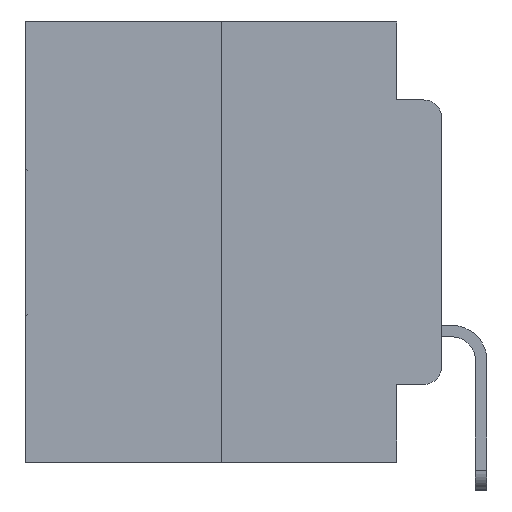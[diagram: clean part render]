
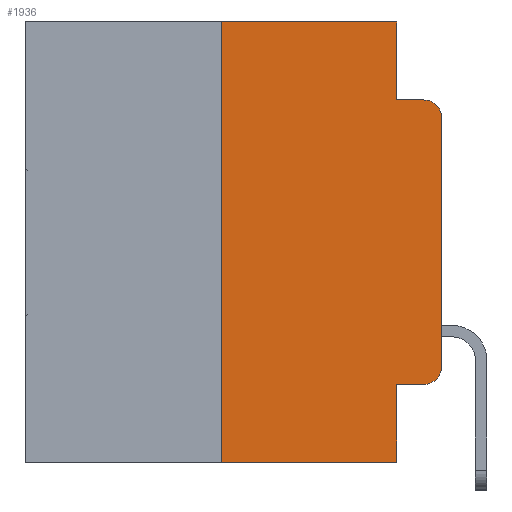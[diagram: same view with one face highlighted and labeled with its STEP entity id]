
A CAD part, left-side view. The second image highlights one B-rep face of the part: STEP entity #1936.
In plain terms, the highlighted planar face has unit normal (-1, 0, 0).
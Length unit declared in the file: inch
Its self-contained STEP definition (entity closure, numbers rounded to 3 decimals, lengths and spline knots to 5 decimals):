
#555 = VERTEX_POINT ( 'NONE', #10674 ) ;
#632 = DIRECTION ( 'NONE',  ( 0., 0., 1. ) ) ;
#837 = DIRECTION ( 'NONE',  ( 0., 0., -1. ) ) ;
#1332 = AXIS2_PLACEMENT_3D ( 'NONE', #7820, #5532, #3255 ) ;
#1486 = DIRECTION ( 'NONE',  ( 0., 0., -1. ) ) ;
#1936 = ADVANCED_FACE ( 'NONE', ( #3103 ), #12876, .F. ) ;
#2161 = AXIS2_PLACEMENT_3D ( 'NONE', #9277, #5025, #837 ) ;
#2241 = ORIENTED_EDGE ( 'NONE', *, *, #6701, .F. ) ;
#2416 = EDGE_CURVE ( 'NONE', #3343, #555, #13606, .T. ) ;
#2468 = DIRECTION ( 'NONE',  ( 0., 0., -1. ) ) ;
#2716 = DIRECTION ( 'NONE',  ( 0., -1., 0. ) ) ;
#3103 = FACE_OUTER_BOUND ( 'NONE', #27822, .T. ) ;
#3255 = DIRECTION ( 'NONE',  ( 0., 0., -1. ) ) ;
#3343 = VERTEX_POINT ( 'NONE', #7509 ) ;
#3593 = DIRECTION ( 'NONE',  ( 0., -1., 0. ) ) ;
#4059 = VECTOR ( 'NONE', #19508, 39.37008 ) ;
#4067 = DIRECTION ( 'NONE',  ( 1., 0., 0. ) ) ;
#4178 = CARTESIAN_POINT ( 'NONE',  ( 0., 0.051, -0.0885 ) ) ;
#4420 = ORIENTED_EDGE ( 'NONE', *, *, #24878, .T. ) ;
#4927 = EDGE_CURVE ( 'NONE', #12223, #23504, #20556, .T. ) ;
#4953 = VERTEX_POINT ( 'NONE', #5848 ) ;
#5025 = DIRECTION ( 'NONE',  ( -1., 0., 0. ) ) ;
#5071 = DIRECTION ( 'NONE',  ( 0., 0., 1. ) ) ;
#5532 = DIRECTION ( 'NONE',  ( -1., 0., 0. ) ) ;
#5848 = CARTESIAN_POINT ( 'NONE',  ( 0., 0.25, -0.5 ) ) ;
#5850 = LINE ( 'NONE', #15894, #25465 ) ;
#6072 = DIRECTION ( 'NONE',  ( 0., 0., -1. ) ) ;
#6505 = LINE ( 'NONE', #15685, #25771 ) ;
#6598 = VECTOR ( 'NONE', #16787, 39.37008 ) ;
#6701 = EDGE_CURVE ( 'NONE', #25876, #19956, #26361, .T. ) ;
#6724 = ORIENTED_EDGE ( 'NONE', *, *, #12757, .F. ) ;
#7311 = VECTOR ( 'NONE', #3593, 39.37008 ) ;
#7509 = CARTESIAN_POINT ( 'NONE',  ( 0., 0.02, -0.4115 ) ) ;
#7820 = CARTESIAN_POINT ( 'NONE',  ( 0., 0.02, -0.3915 ) ) ;
#8266 = CARTESIAN_POINT ( 'NONE',  ( 0., 0.25, 0. ) ) ;
#8915 = CARTESIAN_POINT ( 'NONE',  ( 0., 0.051, 0. ) ) ;
#9277 = CARTESIAN_POINT ( 'NONE',  ( 0., 0.02, -0.1085 ) ) ;
#9475 = CARTESIAN_POINT ( 'NONE',  ( 0., 0.051, -0.0885 ) ) ;
#9565 = EDGE_CURVE ( 'NONE', #17703, #25876, #20539, .T. ) ;
#10046 = CARTESIAN_POINT ( 'NONE',  ( 0., 0.473, -0.5 ) ) ;
#10210 = EDGE_CURVE ( 'NONE', #17473, #17703, #18809, .T. ) ;
#10674 = CARTESIAN_POINT ( 'NONE',  ( 0., 0., -0.3915 ) ) ;
#11434 = ORIENTED_EDGE ( 'NONE', *, *, #20346, .T. ) ;
#12223 = VERTEX_POINT ( 'NONE', #14851 ) ;
#12757 = EDGE_CURVE ( 'NONE', #4953, #17473, #13345, .T. ) ;
#12760 = ORIENTED_EDGE ( 'NONE', *, *, #4927, .F. ) ;
#12876 = PLANE ( 'NONE',  #15464 ) ;
#13345 = LINE ( 'NONE', #8266, #21521 ) ;
#13606 = CIRCLE ( 'NONE', #1332, 0.02 ) ;
#14702 = CARTESIAN_POINT ( 'NONE',  ( 0., 0.473, 0. ) ) ;
#14784 = CARTESIAN_POINT ( 'NONE',  ( 0., 0.051, -0.5 ) ) ;
#14851 = CARTESIAN_POINT ( 'NONE',  ( 0., 0.051, -0.4115 ) ) ;
#15041 = CIRCLE ( 'NONE', #2161, 0.02 ) ;
#15464 = AXIS2_PLACEMENT_3D ( 'NONE', #14702, #4067, #6072 ) ;
#15685 = CARTESIAN_POINT ( 'NONE',  ( 0., 0., 0. ) ) ;
#15763 = CARTESIAN_POINT ( 'NONE',  ( 0., 0., -0.1085 ) ) ;
#15894 = CARTESIAN_POINT ( 'NONE',  ( 0., 0.051, -0.4115 ) ) ;
#16135 = VECTOR ( 'NONE', #2468, 39.37008 ) ;
#16706 = CARTESIAN_POINT ( 'NONE',  ( 0., 0.25, 0. ) ) ;
#16787 = DIRECTION ( 'NONE',  ( 0., -1., 0. ) ) ;
#17473 = VERTEX_POINT ( 'NONE', #16706 ) ;
#17475 = LINE ( 'NONE', #10046, #7311 ) ;
#17703 = VERTEX_POINT ( 'NONE', #27383 ) ;
#17737 = EDGE_CURVE ( 'NONE', #22998, #19956, #15041, .T. ) ;
#18809 = LINE ( 'NONE', #23132, #6598 ) ;
#19508 = DIRECTION ( 'NONE',  ( 0., -1., 0. ) ) ;
#19956 = VERTEX_POINT ( 'NONE', #22729 ) ;
#20030 = ORIENTED_EDGE ( 'NONE', *, *, #24551, .T. ) ;
#20346 = EDGE_CURVE ( 'NONE', #4953, #23504, #17475, .T. ) ;
#20539 = LINE ( 'NONE', #8915, #16135 ) ;
#20556 = LINE ( 'NONE', #23009, #24595 ) ;
#21521 = VECTOR ( 'NONE', #632, 39.37008 ) ;
#22729 = CARTESIAN_POINT ( 'NONE',  ( 0., 0.02, -0.0885 ) ) ;
#22951 = ORIENTED_EDGE ( 'NONE', *, *, #17737, .T. ) ;
#22998 = VERTEX_POINT ( 'NONE', #15763 ) ;
#23009 = CARTESIAN_POINT ( 'NONE',  ( 0., 0.051, 0. ) ) ;
#23132 = CARTESIAN_POINT ( 'NONE',  ( 0., 0.473, 0. ) ) ;
#23504 = VERTEX_POINT ( 'NONE', #14784 ) ;
#24175 = ORIENTED_EDGE ( 'NONE', *, *, #10210, .F. ) ;
#24551 = EDGE_CURVE ( 'NONE', #12223, #3343, #5850, .T. ) ;
#24595 = VECTOR ( 'NONE', #1486, 39.37008 ) ;
#24878 = EDGE_CURVE ( 'NONE', #555, #22998, #6505, .T. ) ;
#25465 = VECTOR ( 'NONE', #2716, 39.37008 ) ;
#25771 = VECTOR ( 'NONE', #5071, 39.37008 ) ;
#25876 = VERTEX_POINT ( 'NONE', #9475 ) ;
#26361 = LINE ( 'NONE', #4178, #4059 ) ;
#26687 = ORIENTED_EDGE ( 'NONE', *, *, #9565, .F. ) ;
#27181 = ORIENTED_EDGE ( 'NONE', *, *, #2416, .T. ) ;
#27383 = CARTESIAN_POINT ( 'NONE',  ( 0., 0.051, 0. ) ) ;
#27822 = EDGE_LOOP ( 'NONE', ( #4420, #22951, #2241, #26687, #24175, #6724, #11434, #12760, #20030, #27181 ) ) ;
